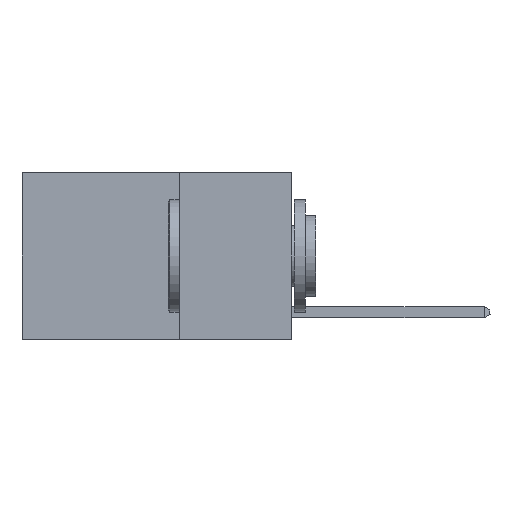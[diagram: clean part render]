
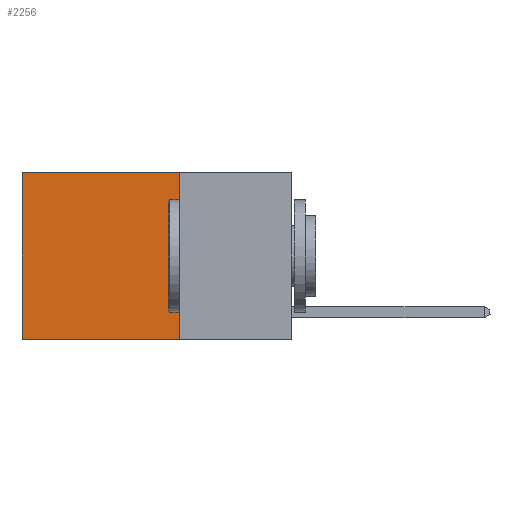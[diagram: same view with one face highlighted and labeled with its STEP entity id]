
A CAD part, left-side view. The second image highlights one B-rep face of the part: STEP entity #2256.
In plain terms, the highlighted planar face has unit normal (-1, 0, 0).
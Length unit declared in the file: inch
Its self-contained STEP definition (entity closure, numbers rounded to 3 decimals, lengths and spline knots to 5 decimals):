
#180 = EDGE_CURVE ( 'NONE', #13006, #10176, #5623, .T. ) ;
#1051 = LINE ( 'NONE', #4171, #1703 ) ;
#1659 = DIRECTION ( 'NONE',  ( 0., 0., -1. ) ) ;
#1660 = DIRECTION ( 'NONE',  ( 0., 0., -1. ) ) ;
#1703 = VECTOR ( 'NONE', #7415, 39.37008 ) ;
#2256 = ADVANCED_FACE ( 'NONE', ( #13311 ), #9743, .F. ) ;
#2403 = ORIENTED_EDGE ( 'NONE', *, *, #12505, .F. ) ;
#2447 = CARTESIAN_POINT ( 'NONE',  ( 0.2625, 0.6, 0. ) ) ;
#3059 = EDGE_CURVE ( 'NONE', #21333, #10034, #19927, .T. ) ;
#3481 = CARTESIAN_POINT ( 'NONE',  ( 0.2625, 0.6, 0. ) ) ;
#3985 = VECTOR ( 'NONE', #1659, 39.37008 ) ;
#4171 = CARTESIAN_POINT ( 'NONE',  ( 0.2625, 0.25, 0. ) ) ;
#4907 = DIRECTION ( 'NONE',  ( 1., 0., 0. ) ) ;
#4934 = CARTESIAN_POINT ( 'NONE',  ( 0.2625, 0.25, -0.37 ) ) ;
#5301 = DIRECTION ( 'NONE',  ( 0., 1., 0. ) ) ;
#5623 = LINE ( 'NONE', #17041, #19229 ) ;
#7415 = DIRECTION ( 'NONE',  ( 0., 0., -1. ) ) ;
#9666 = EDGE_CURVE ( 'NONE', #10176, #10034, #11787, .T. ) ;
#9743 = PLANE ( 'NONE',  #9952 ) ;
#9750 = ORIENTED_EDGE ( 'NONE', *, *, #180, .T. ) ;
#9952 = AXIS2_PLACEMENT_3D ( 'NONE', #10156, #4907, #1660 ) ;
#10034 = VERTEX_POINT ( 'NONE', #11337 ) ;
#10156 = CARTESIAN_POINT ( 'NONE',  ( 0.2625, 0.25, 0. ) ) ;
#10176 = VERTEX_POINT ( 'NONE', #2447 ) ;
#11337 = CARTESIAN_POINT ( 'NONE',  ( 0.2625, 0.6, -0.37 ) ) ;
#11342 = EDGE_LOOP ( 'NONE', ( #18945, #12534, #2403, #9750 ) ) ;
#11787 = LINE ( 'NONE', #3481, #3985 ) ;
#12505 = EDGE_CURVE ( 'NONE', #13006, #21333, #1051, .T. ) ;
#12534 = ORIENTED_EDGE ( 'NONE', *, *, #3059, .F. ) ;
#13006 = VERTEX_POINT ( 'NONE', #20676 ) ;
#13311 = FACE_OUTER_BOUND ( 'NONE', #11342, .T. ) ;
#13542 = CARTESIAN_POINT ( 'NONE',  ( 0.2625, 0.25, -0.37 ) ) ;
#16039 = VECTOR ( 'NONE', #16552, 39.37008 ) ;
#16552 = DIRECTION ( 'NONE',  ( 0., 1., 0. ) ) ;
#17041 = CARTESIAN_POINT ( 'NONE',  ( 0.2625, 0.25, 0. ) ) ;
#18945 = ORIENTED_EDGE ( 'NONE', *, *, #9666, .T. ) ;
#19229 = VECTOR ( 'NONE', #5301, 39.37008 ) ;
#19927 = LINE ( 'NONE', #4934, #16039 ) ;
#20676 = CARTESIAN_POINT ( 'NONE',  ( 0.2625, 0.25, 0. ) ) ;
#21333 = VERTEX_POINT ( 'NONE', #13542 ) ;
